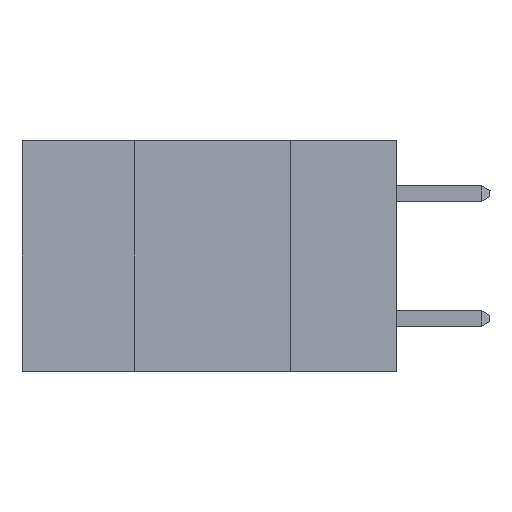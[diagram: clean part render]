
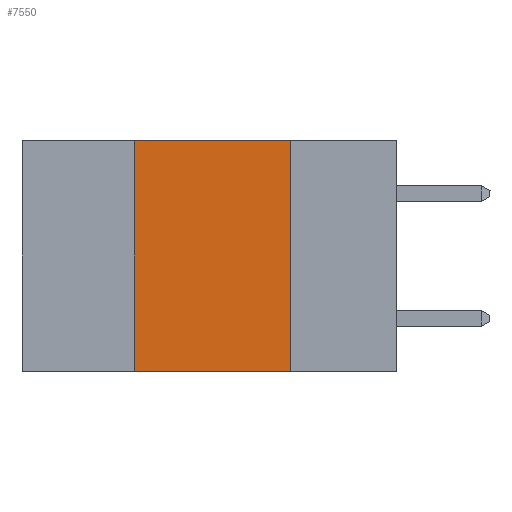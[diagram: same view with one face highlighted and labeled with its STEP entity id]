
A CAD part, left-side view. The second image highlights one B-rep face of the part: STEP entity #7550.
In plain terms, the highlighted planar face has unit normal (-1, 0, 0).
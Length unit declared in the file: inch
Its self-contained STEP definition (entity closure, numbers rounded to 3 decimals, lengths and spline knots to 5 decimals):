
#266 = EDGE_CURVE ( 'NONE', #7251, #5885, #7725, .T. ) ;
#507 = EDGE_LOOP ( 'NONE', ( #2623, #8886, #7581, #6535 ) ) ;
#829 = CARTESIAN_POINT ( 'NONE',  ( 0., 0.6, -0.37 ) ) ;
#849 = VERTEX_POINT ( 'NONE', #8544 ) ;
#1127 = CARTESIAN_POINT ( 'NONE',  ( 0., 0.17, 0. ) ) ;
#2150 = CARTESIAN_POINT ( 'NONE',  ( 0., 0.42, -0.37 ) ) ;
#2537 = EDGE_CURVE ( 'NONE', #5885, #849, #2912, .T. ) ;
#2623 = ORIENTED_EDGE ( 'NONE', *, *, #2537, .F. ) ;
#2912 = LINE ( 'NONE', #1127, #10308 ) ;
#2917 = DIRECTION ( 'NONE',  ( 0., 0., 1. ) ) ;
#3065 = VECTOR ( 'NONE', #8350, 39.37008 ) ;
#3446 = DIRECTION ( 'NONE',  ( 0., 0., -1. ) ) ;
#3627 = DIRECTION ( 'NONE',  ( 0., 0., -1. ) ) ;
#3883 = AXIS2_PLACEMENT_3D ( 'NONE', #4938, #8586, #3446 ) ;
#3957 = CARTESIAN_POINT ( 'NONE',  ( 0., 0.42, 0. ) ) ;
#4515 = VERTEX_POINT ( 'NONE', #2150 ) ;
#4697 = DIRECTION ( 'NONE',  ( 0., -1., 0. ) ) ;
#4938 = CARTESIAN_POINT ( 'NONE',  ( 0., 0.6, 0. ) ) ;
#5280 = LINE ( 'NONE', #829, #3065 ) ;
#5885 = VERTEX_POINT ( 'NONE', #8914 ) ;
#6345 = PLANE ( 'NONE',  #3883 ) ;
#6535 = ORIENTED_EDGE ( 'NONE', *, *, #9754, .T. ) ;
#7251 = VERTEX_POINT ( 'NONE', #7613 ) ;
#7550 = ADVANCED_FACE ( 'NONE', ( #8272 ), #6345, .F. ) ;
#7581 = ORIENTED_EDGE ( 'NONE', *, *, #7594, .F. ) ;
#7594 = EDGE_CURVE ( 'NONE', #4515, #7251, #7756, .T. ) ;
#7613 = CARTESIAN_POINT ( 'NONE',  ( 0., 0.42, 0. ) ) ;
#7725 = LINE ( 'NONE', #8784, #9613 ) ;
#7756 = LINE ( 'NONE', #3957, #9639 ) ;
#8272 = FACE_OUTER_BOUND ( 'NONE', #507, .T. ) ;
#8350 = DIRECTION ( 'NONE',  ( 0., -1., 0. ) ) ;
#8544 = CARTESIAN_POINT ( 'NONE',  ( 0., 0.17, -0.37 ) ) ;
#8586 = DIRECTION ( 'NONE',  ( 1., 0., 0. ) ) ;
#8784 = CARTESIAN_POINT ( 'NONE',  ( 0., 0.6, 0. ) ) ;
#8886 = ORIENTED_EDGE ( 'NONE', *, *, #266, .F. ) ;
#8914 = CARTESIAN_POINT ( 'NONE',  ( 0., 0.17, 0. ) ) ;
#9613 = VECTOR ( 'NONE', #4697, 39.37008 ) ;
#9639 = VECTOR ( 'NONE', #2917, 39.37008 ) ;
#9754 = EDGE_CURVE ( 'NONE', #4515, #849, #5280, .T. ) ;
#10308 = VECTOR ( 'NONE', #3627, 39.37008 ) ;
